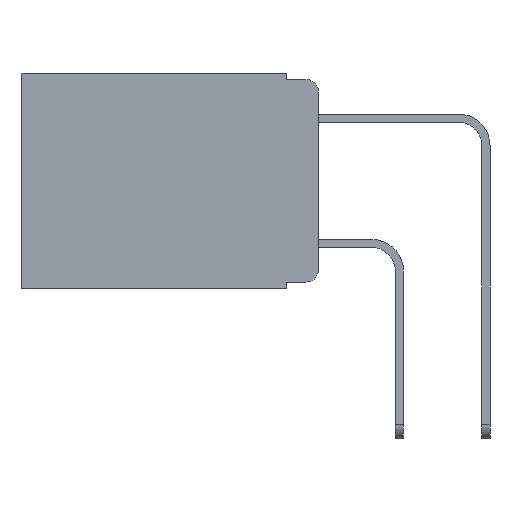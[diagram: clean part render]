
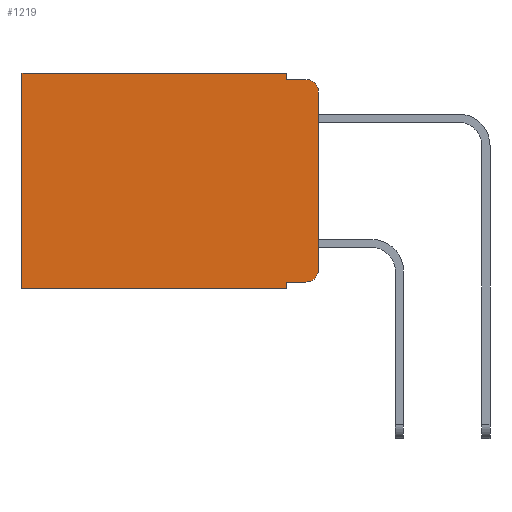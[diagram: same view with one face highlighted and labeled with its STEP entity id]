
A CAD part, left-side view. The second image highlights one B-rep face of the part: STEP entity #1219.
In plain terms, the highlighted planar face has unit normal (-1, 0, 0).
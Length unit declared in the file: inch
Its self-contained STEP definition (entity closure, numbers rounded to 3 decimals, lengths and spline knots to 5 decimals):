
#242 = DIRECTION ( 'NONE',  ( 0., 0., -1. ) ) ;
#287 = VECTOR ( 'NONE', #13178, 39.37008 ) ;
#314 = ORIENTED_EDGE ( 'NONE', *, *, #3403, .T. ) ;
#494 = LINE ( 'NONE', #6267, #3828 ) ;
#512 = ORIENTED_EDGE ( 'NONE', *, *, #12650, .T. ) ;
#865 = CARTESIAN_POINT ( 'NONE',  ( 0.298, 0., -0.343 ) ) ;
#916 = ORIENTED_EDGE ( 'NONE', *, *, #11683, .T. ) ;
#1154 = EDGE_CURVE ( 'NONE', #11747, #11890, #494, .T. ) ;
#1219 = ADVANCED_FACE ( 'NONE', ( #10824 ), #5024, .F. ) ;
#1869 = LINE ( 'NONE', #865, #7041 ) ;
#1893 = DIRECTION ( 'NONE',  ( 0., 0., -1. ) ) ;
#1901 = EDGE_CURVE ( 'NONE', #6793, #6910, #5895, .T. ) ;
#1985 = ORIENTED_EDGE ( 'NONE', *, *, #2662, .F. ) ;
#2145 = VECTOR ( 'NONE', #12310, 39.37008 ) ;
#2636 = VERTEX_POINT ( 'NONE', #12552 ) ;
#2662 = EDGE_CURVE ( 'NONE', #6910, #3535, #10794, .T. ) ;
#3403 = EDGE_CURVE ( 'NONE', #3517, #3535, #12921, .T. ) ;
#3517 = VERTEX_POINT ( 'NONE', #12307 ) ;
#3535 = VERTEX_POINT ( 'NONE', #5676 ) ;
#3744 = CARTESIAN_POINT ( 'NONE',  ( 0.298, 0., 0. ) ) ;
#3757 = AXIS2_PLACEMENT_3D ( 'NONE', #5155, #5090, #5380 ) ;
#3828 = VECTOR ( 'NONE', #242, 39.37008 ) ;
#3996 = CARTESIAN_POINT ( 'NONE',  ( 0.298, 0.02, -0.313 ) ) ;
#4682 = CARTESIAN_POINT ( 'NONE',  ( 0.298, 0., -0.313 ) ) ;
#4801 = AXIS2_PLACEMENT_3D ( 'NONE', #10247, #9703, #9700 ) ;
#4905 = EDGE_CURVE ( 'NONE', #3517, #8759, #7310, .T. ) ;
#5024 = PLANE ( 'NONE',  #3757 ) ;
#5090 = DIRECTION ( 'NONE',  ( 1., 0., 0. ) ) ;
#5126 = DIRECTION ( 'NONE',  ( 0., 0., -1. ) ) ;
#5155 = CARTESIAN_POINT ( 'NONE',  ( 0.298, 0., 0. ) ) ;
#5204 = CARTESIAN_POINT ( 'NONE',  ( 0.298, 0.051, -0.333 ) ) ;
#5380 = DIRECTION ( 'NONE',  ( 0., 0., -1. ) ) ;
#5676 = CARTESIAN_POINT ( 'NONE',  ( 0.298, 0.02, -0.01 ) ) ;
#5895 = LINE ( 'NONE', #11824, #287 ) ;
#6267 = CARTESIAN_POINT ( 'NONE',  ( 0.298, 0.473, 0. ) ) ;
#6661 = CARTESIAN_POINT ( 'NONE',  ( 0.298, 0.051, -0.01 ) ) ;
#6793 = VERTEX_POINT ( 'NONE', #13388 ) ;
#6910 = VERTEX_POINT ( 'NONE', #6661 ) ;
#7041 = VECTOR ( 'NONE', #9490, 39.37008 ) ;
#7177 = VECTOR ( 'NONE', #11679, 39.37008 ) ;
#7310 = LINE ( 'NONE', #3744, #11972 ) ;
#7943 = VECTOR ( 'NONE', #1893, 39.37008 ) ;
#8065 = CARTESIAN_POINT ( 'NONE',  ( 0.298, 0.473, -0.343 ) ) ;
#8467 = CIRCLE ( 'NONE', #10176, 0.02 ) ;
#8759 = VERTEX_POINT ( 'NONE', #4682 ) ;
#8978 = CARTESIAN_POINT ( 'NONE',  ( 0.298, 0.051, -0.333 ) ) ;
#9188 = ORIENTED_EDGE ( 'NONE', *, *, #10848, .F. ) ;
#9404 = CARTESIAN_POINT ( 'NONE',  ( 0.298, 0.051, 0. ) ) ;
#9442 = ORIENTED_EDGE ( 'NONE', *, *, #1154, .T. ) ;
#9490 = DIRECTION ( 'NONE',  ( 0., 1., 0. ) ) ;
#9690 = CARTESIAN_POINT ( 'NONE',  ( 0.298, 0., 0. ) ) ;
#9700 = DIRECTION ( 'NONE',  ( 0., 0., -1. ) ) ;
#9703 = DIRECTION ( 'NONE',  ( -1., 0., 0. ) ) ;
#9774 = CARTESIAN_POINT ( 'NONE',  ( 0.298, 0.473, 0. ) ) ;
#9830 = LINE ( 'NONE', #9690, #7177 ) ;
#10176 = AXIS2_PLACEMENT_3D ( 'NONE', #3996, #11248, #5126 ) ;
#10247 = CARTESIAN_POINT ( 'NONE',  ( 0.298, 0.02, -0.03 ) ) ;
#10279 = ORIENTED_EDGE ( 'NONE', *, *, #13301, .F. ) ;
#10574 = LINE ( 'NONE', #5204, #2145 ) ;
#10768 = DIRECTION ( 'NONE',  ( 0., 0., -1. ) ) ;
#10794 = LINE ( 'NONE', #12705, #11405 ) ;
#10824 = FACE_OUTER_BOUND ( 'NONE', #12987, .T. ) ;
#10848 = EDGE_CURVE ( 'NONE', #2636, #11890, #1869, .T. ) ;
#11041 = ORIENTED_EDGE ( 'NONE', *, *, #1901, .F. ) ;
#11189 = LINE ( 'NONE', #9404, #7943 ) ;
#11248 = DIRECTION ( 'NONE',  ( -1., 0., 0. ) ) ;
#11405 = VECTOR ( 'NONE', #12717, 39.37008 ) ;
#11426 = ORIENTED_EDGE ( 'NONE', *, *, #12008, .T. ) ;
#11679 = DIRECTION ( 'NONE',  ( 0., 1., 0. ) ) ;
#11683 = EDGE_CURVE ( 'NONE', #6793, #11747, #9830, .T. ) ;
#11747 = VERTEX_POINT ( 'NONE', #9774 ) ;
#11824 = CARTESIAN_POINT ( 'NONE',  ( 0.298, 0.051, 0. ) ) ;
#11838 = VERTEX_POINT ( 'NONE', #8978 ) ;
#11890 = VERTEX_POINT ( 'NONE', #8065 ) ;
#11972 = VECTOR ( 'NONE', #10768, 39.37008 ) ;
#12008 = EDGE_CURVE ( 'NONE', #12092, #8759, #8467, .T. ) ;
#12092 = VERTEX_POINT ( 'NONE', #13331 ) ;
#12307 = CARTESIAN_POINT ( 'NONE',  ( 0.298, 0., -0.03 ) ) ;
#12310 = DIRECTION ( 'NONE',  ( 0., -1., 0. ) ) ;
#12552 = CARTESIAN_POINT ( 'NONE',  ( 0.298, 0.051, -0.343 ) ) ;
#12650 = EDGE_CURVE ( 'NONE', #11838, #12092, #10574, .T. ) ;
#12705 = CARTESIAN_POINT ( 'NONE',  ( 0.298, 0.051, -0.01 ) ) ;
#12717 = DIRECTION ( 'NONE',  ( 0., -1., 0. ) ) ;
#12921 = CIRCLE ( 'NONE', #4801, 0.02 ) ;
#12987 = EDGE_LOOP ( 'NONE', ( #13422, #314, #1985, #11041, #916, #9442, #9188, #10279, #512, #11426 ) ) ;
#13178 = DIRECTION ( 'NONE',  ( 0., 0., -1. ) ) ;
#13301 = EDGE_CURVE ( 'NONE', #11838, #2636, #11189, .T. ) ;
#13331 = CARTESIAN_POINT ( 'NONE',  ( 0.298, 0.02, -0.333 ) ) ;
#13388 = CARTESIAN_POINT ( 'NONE',  ( 0.298, 0.051, 0. ) ) ;
#13422 = ORIENTED_EDGE ( 'NONE', *, *, #4905, .F. ) ;
